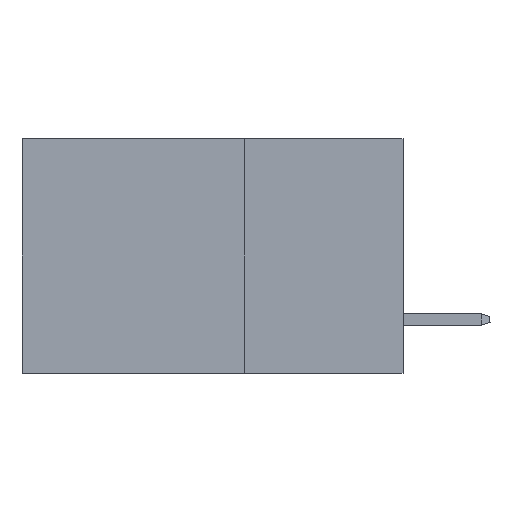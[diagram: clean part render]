
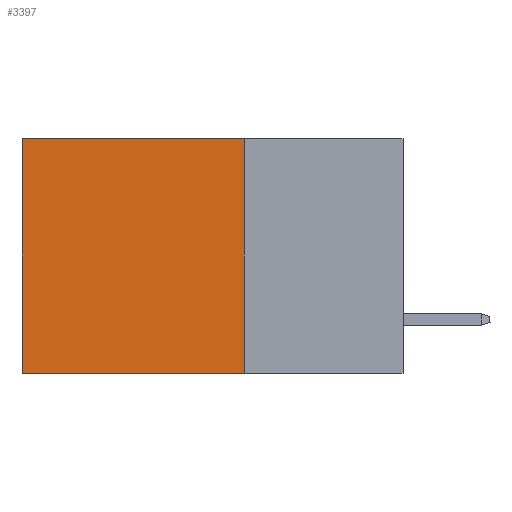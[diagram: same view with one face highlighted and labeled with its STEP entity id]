
A CAD part, left-side view. The second image highlights one B-rep face of the part: STEP entity #3397.
In plain terms, the highlighted planar face has unit normal (-1, 0, 0).
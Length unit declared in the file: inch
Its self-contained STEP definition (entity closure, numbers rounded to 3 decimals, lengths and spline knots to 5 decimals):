
#1169 = CARTESIAN_POINT ( 'NONE',  ( 0.2875, 0.25, 0. ) ) ;
#3397 = ADVANCED_FACE ( 'NONE', ( #6359 ), #4784, .F. ) ;
#3439 = AXIS2_PLACEMENT_3D ( 'NONE', #1169, #18244, #14365 ) ;
#3474 = ORIENTED_EDGE ( 'NONE', *, *, #21195, .F. ) ;
#4190 = CARTESIAN_POINT ( 'NONE',  ( 0.2875, 0.25, -0.37 ) ) ;
#4784 = PLANE ( 'NONE',  #3439 ) ;
#4945 = VERTEX_POINT ( 'NONE', #12558 ) ;
#5318 = CARTESIAN_POINT ( 'NONE',  ( 0.2875, 0.25, 0. ) ) ;
#5798 = VERTEX_POINT ( 'NONE', #4190 ) ;
#6359 = FACE_OUTER_BOUND ( 'NONE', #21622, .T. ) ;
#6465 = ORIENTED_EDGE ( 'NONE', *, *, #21526, .T. ) ;
#7373 = VERTEX_POINT ( 'NONE', #17618 ) ;
#7991 = LINE ( 'NONE', #19497, #18970 ) ;
#8759 = LINE ( 'NONE', #5318, #18986 ) ;
#8771 = VECTOR ( 'NONE', #17163, 39.37008 ) ;
#10183 = DIRECTION ( 'NONE',  ( 0., 1., 0. ) ) ;
#11375 = LINE ( 'NONE', #16530, #12293 ) ;
#12293 = VECTOR ( 'NONE', #13118, 39.37008 ) ;
#12490 = ORIENTED_EDGE ( 'NONE', *, *, #21334, .F. ) ;
#12558 = CARTESIAN_POINT ( 'NONE',  ( 0.2875, 0.6, 0. ) ) ;
#12958 = CARTESIAN_POINT ( 'NONE',  ( 0.2875, 0.25, 0. ) ) ;
#13118 = DIRECTION ( 'NONE',  ( 0., 1., 0. ) ) ;
#14365 = DIRECTION ( 'NONE',  ( 0., 0., -1. ) ) ;
#15604 = LINE ( 'NONE', #17388, #8771 ) ;
#16101 = ORIENTED_EDGE ( 'NONE', *, *, #17774, .T. ) ;
#16530 = CARTESIAN_POINT ( 'NONE',  ( 0.2875, 0.25, -0.37 ) ) ;
#17163 = DIRECTION ( 'NONE',  ( 0., 0., -1. ) ) ;
#17388 = CARTESIAN_POINT ( 'NONE',  ( 0.2875, 0.6, 0. ) ) ;
#17618 = CARTESIAN_POINT ( 'NONE',  ( 0.2875, 0.6, -0.37 ) ) ;
#17774 = EDGE_CURVE ( 'NONE', #4945, #7373, #15604, .T. ) ;
#18201 = DIRECTION ( 'NONE',  ( 0., 0., -1. ) ) ;
#18244 = DIRECTION ( 'NONE',  ( 1., 0., 0. ) ) ;
#18714 = VERTEX_POINT ( 'NONE', #12958 ) ;
#18970 = VECTOR ( 'NONE', #18201, 39.37008 ) ;
#18986 = VECTOR ( 'NONE', #10183, 39.37008 ) ;
#19497 = CARTESIAN_POINT ( 'NONE',  ( 0.2875, 0.25, 0. ) ) ;
#21195 = EDGE_CURVE ( 'NONE', #18714, #5798, #7991, .T. ) ;
#21334 = EDGE_CURVE ( 'NONE', #5798, #7373, #11375, .T. ) ;
#21526 = EDGE_CURVE ( 'NONE', #18714, #4945, #8759, .T. ) ;
#21622 = EDGE_LOOP ( 'NONE', ( #16101, #12490, #3474, #6465 ) ) ;
